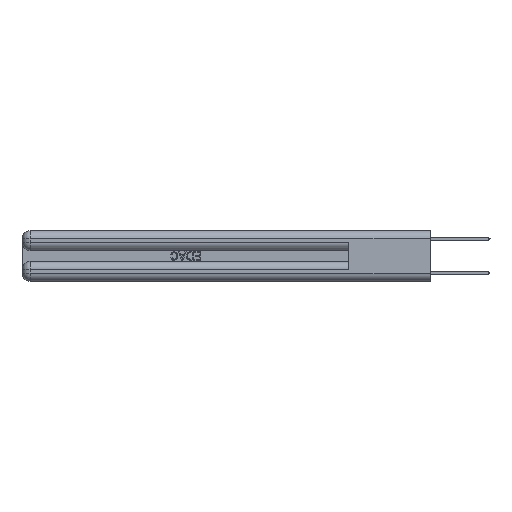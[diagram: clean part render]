
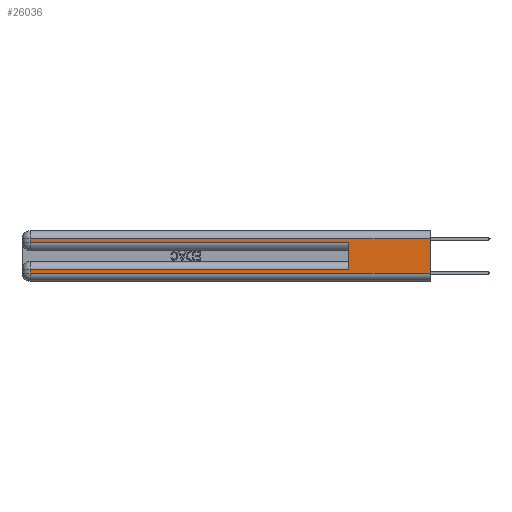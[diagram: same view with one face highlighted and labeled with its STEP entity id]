
A CAD part, left-side view. The second image highlights one B-rep face of the part: STEP entity #26036.
In plain terms, the highlighted planar face has unit normal (-1, 0, 0).
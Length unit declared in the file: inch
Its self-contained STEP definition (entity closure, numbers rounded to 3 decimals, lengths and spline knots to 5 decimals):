
#1373 = LINE ( 'NONE', #15485, #17143 ) ;
#2396 = CARTESIAN_POINT ( 'NONE',  ( 0., 0.6, 0.085 ) ) ;
#2641 = ORIENTED_EDGE ( 'NONE', *, *, #8728, .T. ) ;
#2916 = DIRECTION ( 'NONE',  ( 0., 0., -1. ) ) ;
#3405 = DIRECTION ( 'NONE',  ( 0., 0., 1. ) ) ;
#4007 = LINE ( 'NONE', #29632, #8472 ) ;
#4089 = EDGE_CURVE ( 'NONE', #8592, #22638, #1373, .T. ) ;
#5159 = EDGE_CURVE ( 'NONE', #8851, #23701, #20364, .T. ) ;
#5169 = LINE ( 'NONE', #14263, #12005 ) ;
#5389 = CARTESIAN_POINT ( 'NONE',  ( 0., 0., 0.285 ) ) ;
#5710 = LINE ( 'NONE', #24189, #7635 ) ;
#6012 = EDGE_CURVE ( 'NONE', #21622, #8592, #13331, .T. ) ;
#6140 = VERTEX_POINT ( 'NONE', #17048 ) ;
#6875 = CARTESIAN_POINT ( 'NONE',  ( 0., 2.94, 0.37 ) ) ;
#7615 = DIRECTION ( 'NONE',  ( 0., -1., 0. ) ) ;
#7635 = VECTOR ( 'NONE', #3405, 39.37008 ) ;
#8472 = VECTOR ( 'NONE', #27207, 39.37008 ) ;
#8592 = VERTEX_POINT ( 'NONE', #16384 ) ;
#8728 = EDGE_CURVE ( 'NONE', #22638, #18643, #24410, .T. ) ;
#8851 = VERTEX_POINT ( 'NONE', #26849 ) ;
#9141 = EDGE_LOOP ( 'NONE', ( #11737, #28083, #18480, #24281, #15713, #24143, #23092, #2641 ) ) ;
#10108 = DIRECTION ( 'NONE',  ( 0., -1., 0. ) ) ;
#11271 = VECTOR ( 'NONE', #7615, 39.37008 ) ;
#11737 = ORIENTED_EDGE ( 'NONE', *, *, #20027, .F. ) ;
#12005 = VECTOR ( 'NONE', #19121, 39.37008 ) ;
#12074 = LINE ( 'NONE', #5389, #14570 ) ;
#12357 = CARTESIAN_POINT ( 'NONE',  ( 0., 0., 0.37 ) ) ;
#12598 = AXIS2_PLACEMENT_3D ( 'NONE', #12357, #16887, #2916 ) ;
#13247 = EDGE_CURVE ( 'NONE', #22863, #8851, #4007, .T. ) ;
#13331 = LINE ( 'NONE', #29415, #19193 ) ;
#13540 = DIRECTION ( 'NONE',  ( 0., 0., -1. ) ) ;
#14263 = CARTESIAN_POINT ( 'NONE',  ( 0., 0., 0.37 ) ) ;
#14570 = VECTOR ( 'NONE', #10108, 39.37008 ) ;
#15485 = CARTESIAN_POINT ( 'NONE',  ( 0., 2.94, 0.37 ) ) ;
#15713 = ORIENTED_EDGE ( 'NONE', *, *, #16428, .F. ) ;
#16384 = CARTESIAN_POINT ( 'NONE',  ( 0., 2.94, 0.085 ) ) ;
#16428 = EDGE_CURVE ( 'NONE', #21622, #6140, #5710, .T. ) ;
#16439 = PLANE ( 'NONE',  #12598 ) ;
#16887 = DIRECTION ( 'NONE',  ( 1., 0., 0. ) ) ;
#17048 = CARTESIAN_POINT ( 'NONE',  ( 0., 0.6, 0.285 ) ) ;
#17143 = VECTOR ( 'NONE', #24727, 39.37008 ) ;
#18480 = ORIENTED_EDGE ( 'NONE', *, *, #5159, .T. ) ;
#18587 = FACE_OUTER_BOUND ( 'NONE', #9141, .T. ) ;
#18643 = VERTEX_POINT ( 'NONE', #25282 ) ;
#19121 = DIRECTION ( 'NONE',  ( 0., 0., -1. ) ) ;
#19193 = VECTOR ( 'NONE', #27114, 39.37008 ) ;
#20027 = EDGE_CURVE ( 'NONE', #22863, #18643, #5169, .T. ) ;
#20364 = LINE ( 'NONE', #6875, #27835 ) ;
#21622 = VERTEX_POINT ( 'NONE', #2396 ) ;
#21844 = CARTESIAN_POINT ( 'NONE',  ( 0., 0., 0.06 ) ) ;
#22638 = VERTEX_POINT ( 'NONE', #28682 ) ;
#22863 = VERTEX_POINT ( 'NONE', #23040 ) ;
#23040 = CARTESIAN_POINT ( 'NONE',  ( 0., 0., 0.31 ) ) ;
#23092 = ORIENTED_EDGE ( 'NONE', *, *, #4089, .T. ) ;
#23701 = VERTEX_POINT ( 'NONE', #27077 ) ;
#24143 = ORIENTED_EDGE ( 'NONE', *, *, #6012, .T. ) ;
#24189 = CARTESIAN_POINT ( 'NONE',  ( 0., 0.6, 0.145 ) ) ;
#24281 = ORIENTED_EDGE ( 'NONE', *, *, #27254, .T. ) ;
#24410 = LINE ( 'NONE', #21844, #11271 ) ;
#24727 = DIRECTION ( 'NONE',  ( 0., 0., -1. ) ) ;
#25282 = CARTESIAN_POINT ( 'NONE',  ( 0., 0., 0.06 ) ) ;
#26036 = ADVANCED_FACE ( 'NONE', ( #18587 ), #16439, .F. ) ;
#26849 = CARTESIAN_POINT ( 'NONE',  ( 0., 2.94, 0.31 ) ) ;
#27077 = CARTESIAN_POINT ( 'NONE',  ( 0., 2.94, 0.285 ) ) ;
#27114 = DIRECTION ( 'NONE',  ( 0., 1., 0. ) ) ;
#27207 = DIRECTION ( 'NONE',  ( 0., 1., 0. ) ) ;
#27254 = EDGE_CURVE ( 'NONE', #23701, #6140, #12074, .T. ) ;
#27835 = VECTOR ( 'NONE', #13540, 39.37008 ) ;
#28083 = ORIENTED_EDGE ( 'NONE', *, *, #13247, .T. ) ;
#28682 = CARTESIAN_POINT ( 'NONE',  ( 0., 2.94, 0.06 ) ) ;
#29415 = CARTESIAN_POINT ( 'NONE',  ( 0., 0., 0.085 ) ) ;
#29632 = CARTESIAN_POINT ( 'NONE',  ( 0., 0., 0.31 ) ) ;
